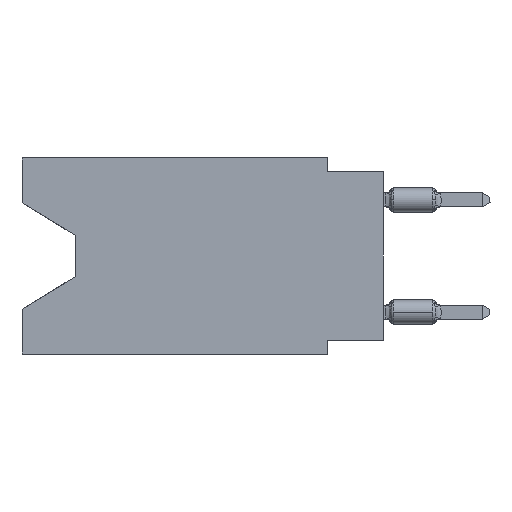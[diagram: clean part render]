
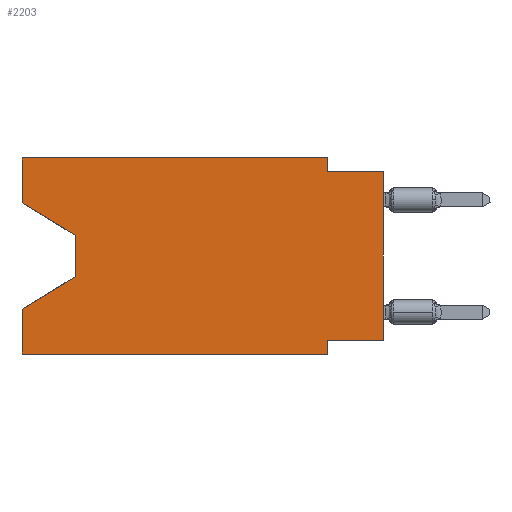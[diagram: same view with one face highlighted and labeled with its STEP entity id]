
A CAD part, left-side view. The second image highlights one B-rep face of the part: STEP entity #2203.
In plain terms, the highlighted planar face has unit normal (-1, 0, 0).
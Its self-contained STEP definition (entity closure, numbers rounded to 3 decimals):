
#149 = ORIENTED_EDGE ( 'NONE', *, *, #11184, .T. ) ;
#1156 = LINE ( 'NONE', #45917, #9653 ) ;
#1334 = PLANE ( 'NONE',  #20585 ) ;
#2203 = ADVANCED_FACE ( 'NONE', ( #13613 ), #1334, .F. ) ;
#2365 = CARTESIAN_POINT ( 'NONE',  ( 0., 2.54, -8.89 ) ) ;
#2621 = EDGE_CURVE ( 'NONE', #46105, #4318, #22339, .T. ) ;
#3563 = CARTESIAN_POINT ( 'NONE',  ( 0., 16.383, -8.89 ) ) ;
#3986 = EDGE_CURVE ( 'NONE', #47961, #4318, #31263, .T. ) ;
#4318 = VERTEX_POINT ( 'NONE', #47887 ) ;
#4913 = CARTESIAN_POINT ( 'NONE',  ( 0., 13.97, -5.385 ) ) ;
#4965 = DIRECTION ( 'NONE',  ( 0., -1., 0. ) ) ;
#5314 = LINE ( 'NONE', #6173, #41296 ) ;
#6173 = CARTESIAN_POINT ( 'NONE',  ( 0., 16.383, -8.89 ) ) ;
#6268 = LINE ( 'NONE', #32330, #25895 ) ;
#6532 = CARTESIAN_POINT ( 'NONE',  ( 0., 2.54, -0.635 ) ) ;
#6852 = LINE ( 'NONE', #10678, #34751 ) ;
#7034 = DIRECTION ( 'NONE',  ( 0., 0., 1. ) ) ;
#8098 = DIRECTION ( 'NONE',  ( 0., -1., 0. ) ) ;
#8895 = VERTEX_POINT ( 'NONE', #47594 ) ;
#9356 = LINE ( 'NONE', #45070, #54195 ) ;
#9653 = VECTOR ( 'NONE', #46203, 1000. ) ;
#9779 = ORIENTED_EDGE ( 'NONE', *, *, #42218, .T. ) ;
#10105 = DIRECTION ( 'NONE',  ( 0., 0., -1. ) ) ;
#10401 = ORIENTED_EDGE ( 'NONE', *, *, #19650, .F. ) ;
#10678 = CARTESIAN_POINT ( 'NONE',  ( 0., 2.54, 0. ) ) ;
#11184 = EDGE_CURVE ( 'NONE', #46546, #47961, #6268, .T. ) ;
#11305 = ORIENTED_EDGE ( 'NONE', *, *, #3986, .T. ) ;
#12268 = ORIENTED_EDGE ( 'NONE', *, *, #45436, .T. ) ;
#12303 = VERTEX_POINT ( 'NONE', #2365 ) ;
#13564 = EDGE_CURVE ( 'NONE', #8895, #21265, #37775, .T. ) ;
#13613 = FACE_OUTER_BOUND ( 'NONE', #50834, .T. ) ;
#13753 = CARTESIAN_POINT ( 'NONE',  ( 0., 2.54, -8.255 ) ) ;
#13845 = CARTESIAN_POINT ( 'NONE',  ( 0., 16.383, 0. ) ) ;
#15490 = CARTESIAN_POINT ( 'NONE',  ( 0., 13.97, -3.505 ) ) ;
#17967 = ORIENTED_EDGE ( 'NONE', *, *, #53182, .F. ) ;
#18008 = CARTESIAN_POINT ( 'NONE',  ( 0., 16.383, -2.038 ) ) ;
#19370 = VERTEX_POINT ( 'NONE', #6532 ) ;
#19650 = EDGE_CURVE ( 'NONE', #8895, #56068, #1156, .T. ) ;
#20195 = CARTESIAN_POINT ( 'NONE',  ( 0., 0., 0. ) ) ;
#20585 = AXIS2_PLACEMENT_3D ( 'NONE', #49353, #32069, #50225 ) ;
#20879 = DIRECTION ( 'NONE',  ( 0., 0., -1. ) ) ;
#21265 = VERTEX_POINT ( 'NONE', #29474 ) ;
#22339 = LINE ( 'NONE', #13845, #48732 ) ;
#24315 = EDGE_CURVE ( 'NONE', #55206, #39104, #9356, .T. ) ;
#25788 = VECTOR ( 'NONE', #48761, 1000. ) ;
#25895 = VECTOR ( 'NONE', #32628, 1000. ) ;
#28384 = VECTOR ( 'NONE', #7034, 1000. ) ;
#28867 = EDGE_CURVE ( 'NONE', #39104, #19370, #6852, .T. ) ;
#29474 = CARTESIAN_POINT ( 'NONE',  ( 0., 0., -0.635 ) ) ;
#31263 = LINE ( 'NONE', #4913, #42243 ) ;
#32069 = DIRECTION ( 'NONE',  ( 1., 0., 0. ) ) ;
#32330 = CARTESIAN_POINT ( 'NONE',  ( 0., 13.97, -3.505 ) ) ;
#32540 = DIRECTION ( 'NONE',  ( 0., -1., 0. ) ) ;
#32628 = DIRECTION ( 'NONE',  ( 0., 0., -1. ) ) ;
#33213 = VECTOR ( 'NONE', #8098, 1000. ) ;
#33496 = CARTESIAN_POINT ( 'NONE',  ( 0., 2.54, -8.89 ) ) ;
#34062 = ORIENTED_EDGE ( 'NONE', *, *, #2621, .F. ) ;
#34421 = ORIENTED_EDGE ( 'NONE', *, *, #41213, .F. ) ;
#34751 = VECTOR ( 'NONE', #10105, 1000. ) ;
#35574 = LINE ( 'NONE', #18008, #25788 ) ;
#35848 = CARTESIAN_POINT ( 'NONE',  ( 0., 16.383, 0. ) ) ;
#36045 = EDGE_CURVE ( 'NONE', #48734, #55206, #45708, .T. ) ;
#37775 = LINE ( 'NONE', #20195, #28384 ) ;
#38822 = LINE ( 'NONE', #56714, #33213 ) ;
#39104 = VERTEX_POINT ( 'NONE', #43941 ) ;
#41033 = CARTESIAN_POINT ( 'NONE',  ( 0., 16.383, 0. ) ) ;
#41213 = EDGE_CURVE ( 'NONE', #19370, #21265, #38822, .T. ) ;
#41296 = VECTOR ( 'NONE', #32540, 1000. ) ;
#41355 = DIRECTION ( 'NONE',  ( 0., 0., 1. ) ) ;
#42156 = VECTOR ( 'NONE', #20879, 1000. ) ;
#42218 = EDGE_CURVE ( 'NONE', #46105, #12303, #5314, .T. ) ;
#42243 = VECTOR ( 'NONE', #50289, 1000. ) ;
#43415 = LINE ( 'NONE', #33496, #42156 ) ;
#43505 = ORIENTED_EDGE ( 'NONE', *, *, #13564, .T. ) ;
#43941 = CARTESIAN_POINT ( 'NONE',  ( 0., 2.54, 0. ) ) ;
#45070 = CARTESIAN_POINT ( 'NONE',  ( 0., 16.383, 0. ) ) ;
#45436 = EDGE_CURVE ( 'NONE', #48734, #46546, #35574, .T. ) ;
#45610 = ORIENTED_EDGE ( 'NONE', *, *, #28867, .F. ) ;
#45708 = LINE ( 'NONE', #41033, #48309 ) ;
#45917 = CARTESIAN_POINT ( 'NONE',  ( 0., 0., -8.255 ) ) ;
#46105 = VERTEX_POINT ( 'NONE', #3563 ) ;
#46203 = DIRECTION ( 'NONE',  ( 0., 1., 0. ) ) ;
#46546 = VERTEX_POINT ( 'NONE', #15490 ) ;
#47594 = CARTESIAN_POINT ( 'NONE',  ( 0., 0., -8.255 ) ) ;
#47794 = CARTESIAN_POINT ( 'NONE',  ( 0., 16.383, -2.038 ) ) ;
#47887 = CARTESIAN_POINT ( 'NONE',  ( 0., 16.383, -6.852 ) ) ;
#47961 = VERTEX_POINT ( 'NONE', #55950 ) ;
#48309 = VECTOR ( 'NONE', #54230, 1000. ) ;
#48732 = VECTOR ( 'NONE', #41355, 1000. ) ;
#48734 = VERTEX_POINT ( 'NONE', #47794 ) ;
#48761 = DIRECTION ( 'NONE',  ( 0., -0.855, -0.519 ) ) ;
#49290 = ORIENTED_EDGE ( 'NONE', *, *, #24315, .F. ) ;
#49353 = CARTESIAN_POINT ( 'NONE',  ( 0., 16.383, 0. ) ) ;
#50225 = DIRECTION ( 'NONE',  ( 0., 0., -1. ) ) ;
#50289 = DIRECTION ( 'NONE',  ( 0., 0.855, -0.519 ) ) ;
#50834 = EDGE_LOOP ( 'NONE', ( #12268, #149, #11305, #34062, #9779, #17967, #10401, #43505, #34421, #45610, #49290, #55490 ) ) ;
#53182 = EDGE_CURVE ( 'NONE', #56068, #12303, #43415, .T. ) ;
#54195 = VECTOR ( 'NONE', #4965, 1000. ) ;
#54230 = DIRECTION ( 'NONE',  ( 0., 0., 1. ) ) ;
#55206 = VERTEX_POINT ( 'NONE', #35848 ) ;
#55490 = ORIENTED_EDGE ( 'NONE', *, *, #36045, .F. ) ;
#55950 = CARTESIAN_POINT ( 'NONE',  ( 0., 13.97, -5.385 ) ) ;
#56068 = VERTEX_POINT ( 'NONE', #13753 ) ;
#56714 = CARTESIAN_POINT ( 'NONE',  ( 0., 0., -0.635 ) ) ;
